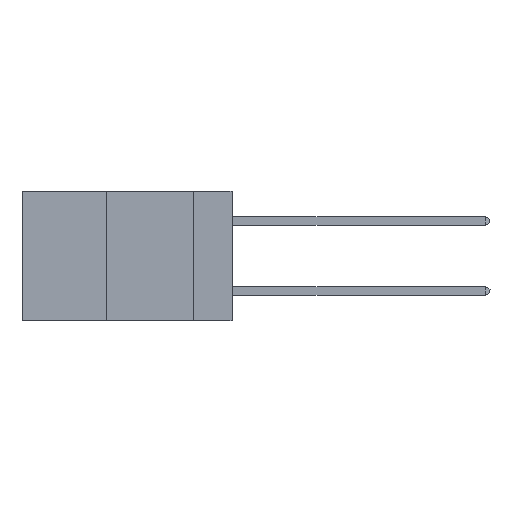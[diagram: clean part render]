
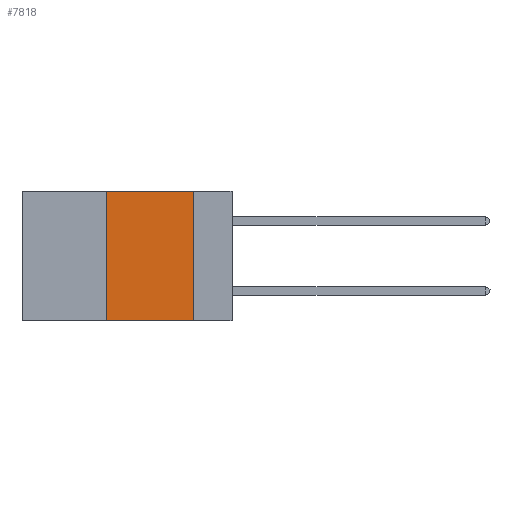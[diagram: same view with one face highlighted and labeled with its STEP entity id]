
A CAD part, left-side view. The second image highlights one B-rep face of the part: STEP entity #7818.
In plain terms, the highlighted planar face has unit normal (-1, 0, 0).
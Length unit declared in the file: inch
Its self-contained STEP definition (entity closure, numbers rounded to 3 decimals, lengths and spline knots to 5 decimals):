
#1010 = LINE ( 'NONE', #17989, #10607 ) ;
#1363 = EDGE_CURVE ( 'NONE', #3770, #4862, #1010, .T. ) ;
#1983 = VERTEX_POINT ( 'NONE', #8521 ) ;
#3011 = VECTOR ( 'NONE', #11315, 39.37008 ) ;
#3405 = VECTOR ( 'NONE', #4126, 39.37008 ) ;
#3416 = DIRECTION ( 'NONE',  ( 0., 0., 1. ) ) ;
#3623 = DIRECTION ( 'NONE',  ( 1., 0., 0. ) ) ;
#3770 = VERTEX_POINT ( 'NONE', #15351 ) ;
#4126 = DIRECTION ( 'NONE',  ( 0., -1., 0. ) ) ;
#4320 = CARTESIAN_POINT ( 'NONE',  ( 0., 0.6, -0.37 ) ) ;
#4434 = FACE_OUTER_BOUND ( 'NONE', #13830, .T. ) ;
#4862 = VERTEX_POINT ( 'NONE', #14874 ) ;
#5322 = ORIENTED_EDGE ( 'NONE', *, *, #15607, .F. ) ;
#5588 = VERTEX_POINT ( 'NONE', #11461 ) ;
#6391 = CARTESIAN_POINT ( 'NONE',  ( 0., 0.36, 0. ) ) ;
#6835 = ORIENTED_EDGE ( 'NONE', *, *, #7142, .F. ) ;
#7142 = EDGE_CURVE ( 'NONE', #1983, #3770, #14890, .T. ) ;
#7818 = ADVANCED_FACE ( 'NONE', ( #4434 ), #9481, .F. ) ;
#8521 = CARTESIAN_POINT ( 'NONE',  ( 0., 0.36, -0.37 ) ) ;
#8946 = LINE ( 'NONE', #4320, #3405 ) ;
#9441 = LINE ( 'NONE', #15656, #3011 ) ;
#9481 = PLANE ( 'NONE',  #13167 ) ;
#9971 = EDGE_CURVE ( 'NONE', #1983, #5588, #8946, .T. ) ;
#10130 = ORIENTED_EDGE ( 'NONE', *, *, #9971, .T. ) ;
#10607 = VECTOR ( 'NONE', #13738, 39.37008 ) ;
#10918 = CARTESIAN_POINT ( 'NONE',  ( 0., 0.6, 0. ) ) ;
#11315 = DIRECTION ( 'NONE',  ( 0., 0., -1. ) ) ;
#11461 = CARTESIAN_POINT ( 'NONE',  ( 0., 0.11, -0.37 ) ) ;
#13167 = AXIS2_PLACEMENT_3D ( 'NONE', #10918, #3623, #13833 ) ;
#13738 = DIRECTION ( 'NONE',  ( 0., -1., 0. ) ) ;
#13830 = EDGE_LOOP ( 'NONE', ( #5322, #14249, #6835, #10130 ) ) ;
#13833 = DIRECTION ( 'NONE',  ( 0., 0., -1. ) ) ;
#14249 = ORIENTED_EDGE ( 'NONE', *, *, #1363, .F. ) ;
#14874 = CARTESIAN_POINT ( 'NONE',  ( 0., 0.11, 0. ) ) ;
#14890 = LINE ( 'NONE', #6391, #15566 ) ;
#15351 = CARTESIAN_POINT ( 'NONE',  ( 0., 0.36, 0. ) ) ;
#15566 = VECTOR ( 'NONE', #3416, 39.37008 ) ;
#15607 = EDGE_CURVE ( 'NONE', #4862, #5588, #9441, .T. ) ;
#15656 = CARTESIAN_POINT ( 'NONE',  ( 0., 0.11, 0. ) ) ;
#17989 = CARTESIAN_POINT ( 'NONE',  ( 0., 0.6, 0. ) ) ;
